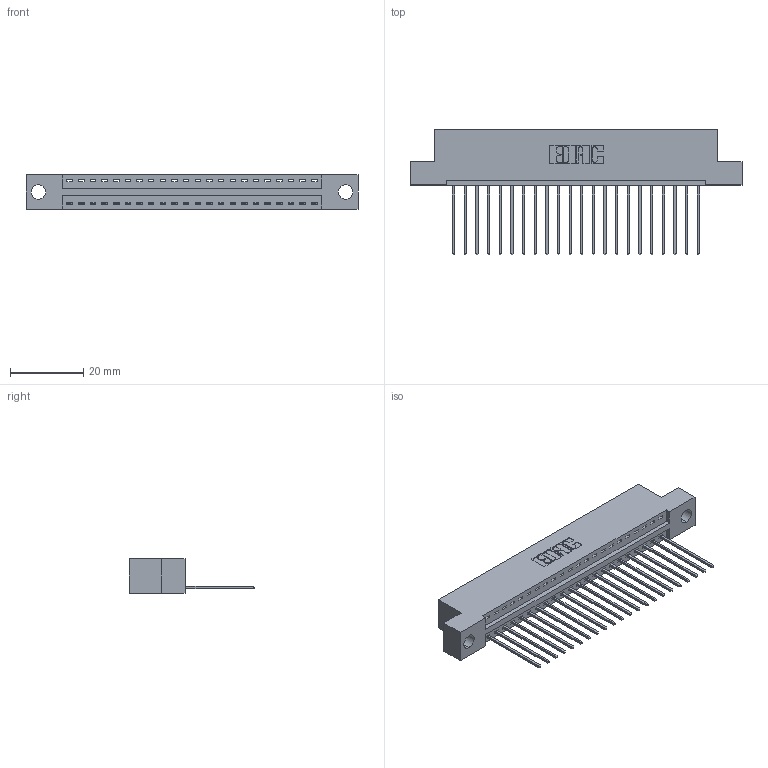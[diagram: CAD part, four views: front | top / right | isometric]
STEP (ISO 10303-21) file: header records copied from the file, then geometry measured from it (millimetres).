
FILE_DESCRIPTION (( 'STEP AP203' ), '1' );
FILE_NAME ('346-022-541-104.STEP', '2022-05-05T19:54:25', ( '' ), ( '' ), 'SwSTEP 2.0', 'SolidWorks 2020', '' );
FILE_SCHEMA (( 'CONFIG_CONTROL_DESIGN' ));
Length unit declared in the file: inch
Products named in the file (3): 346 Part_Flush Mounting Lugs - 0.156 Dia-TH; 346-022-541-104; 345-292-001_345-293-141
Assembly tree (23 placements, depth 2):
  346-022-541-104
    346 Part_Flush Mounting Lugs - 0.156 Dia-TH
    345-292-001_345-293-141  x22
Bounding box: 90.42 x 34.29 x 9.4 mm (x, y, z)
Volume: 8484.4 mm3; surface area: 10659.6 mm2
Topology: 23 solids, 23 shells, 1412 faces, 4237 edges, 2794 vertices
Faces by surface type: plane 970, cylinder 442
Entity records: 16783 total; most frequent: CARTESIAN_POINT 2892, ORIENTED_EDGE 2846, DIRECTION 2575, EDGE_CURVE 1423, LINE 1203, VECTOR 1203, VERTEX_POINT 946, AXIS2_PLACEMENT_3D 686
